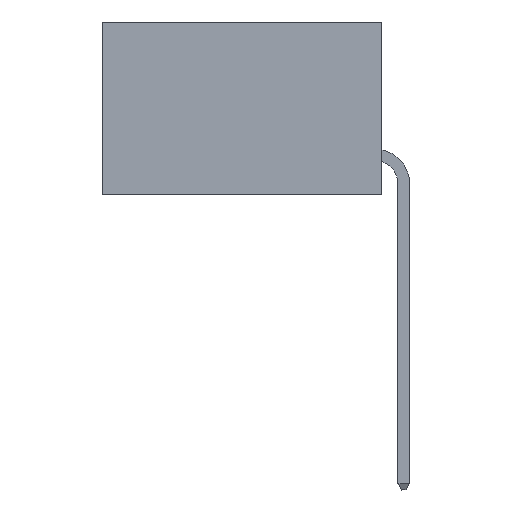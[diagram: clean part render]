
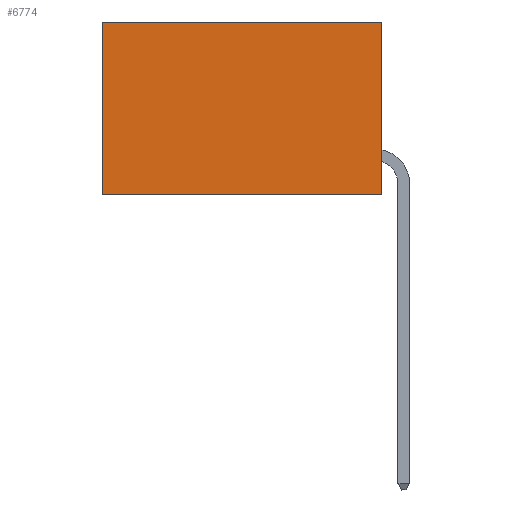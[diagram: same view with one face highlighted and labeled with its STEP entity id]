
A CAD part, left-side view. The second image highlights one B-rep face of the part: STEP entity #6774.
In plain terms, the highlighted planar face has unit normal (-1, 0, 0).
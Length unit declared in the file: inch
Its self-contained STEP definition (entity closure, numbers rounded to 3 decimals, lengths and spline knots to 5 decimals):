
#1500 = VECTOR ( 'NONE', #10096, 39.37008 ) ;
#1621 = CARTESIAN_POINT ( 'NONE',  ( 0.2875, 0.6, 0. ) ) ;
#1684 = CARTESIAN_POINT ( 'NONE',  ( 0.2875, 0., 0. ) ) ;
#2334 = CARTESIAN_POINT ( 'NONE',  ( 0.2875, 0., 0. ) ) ;
#2778 = ORIENTED_EDGE ( 'NONE', *, *, #13709, .F. ) ;
#3225 = DIRECTION ( 'NONE',  ( 0., 0., -1. ) ) ;
#3519 = PLANE ( 'NONE',  #7349 ) ;
#3850 = LINE ( 'NONE', #5357, #6901 ) ;
#4178 = ORIENTED_EDGE ( 'NONE', *, *, #12135, .T. ) ;
#4188 = VERTEX_POINT ( 'NONE', #7121 ) ;
#4254 = EDGE_LOOP ( 'NONE', ( #4178, #9367, #2778, #13090 ) ) ;
#5253 = VECTOR ( 'NONE', #8960, 39.37008 ) ;
#5357 = CARTESIAN_POINT ( 'NONE',  ( 0.2875, 0., 0. ) ) ;
#5642 = CARTESIAN_POINT ( 'NONE',  ( 0.2875, 0., 0. ) ) ;
#5748 = CARTESIAN_POINT ( 'NONE',  ( 0.2875, 0., -0.37 ) ) ;
#6328 = VECTOR ( 'NONE', #7014, 39.37008 ) ;
#6774 = ADVANCED_FACE ( 'NONE', ( #6978 ), #3519, .F. ) ;
#6892 = VERTEX_POINT ( 'NONE', #1684 ) ;
#6901 = VECTOR ( 'NONE', #3225, 39.37008 ) ;
#6978 = FACE_OUTER_BOUND ( 'NONE', #4254, .T. ) ;
#7014 = DIRECTION ( 'NONE',  ( 0., 0., -1. ) ) ;
#7121 = CARTESIAN_POINT ( 'NONE',  ( 0.2875, 0., -0.37 ) ) ;
#7349 = AXIS2_PLACEMENT_3D ( 'NONE', #2334, #12230, #11014 ) ;
#7604 = LINE ( 'NONE', #5748, #1500 ) ;
#8324 = EDGE_CURVE ( 'NONE', #6892, #10423, #13953, .T. ) ;
#8960 = DIRECTION ( 'NONE',  ( 0., 1., 0. ) ) ;
#9367 = ORIENTED_EDGE ( 'NONE', *, *, #13352, .F. ) ;
#9400 = CARTESIAN_POINT ( 'NONE',  ( 0.2875, 0.6, -0.37 ) ) ;
#10096 = DIRECTION ( 'NONE',  ( 0., 1., 0. ) ) ;
#10255 = LINE ( 'NONE', #1621, #6328 ) ;
#10423 = VERTEX_POINT ( 'NONE', #11008 ) ;
#11008 = CARTESIAN_POINT ( 'NONE',  ( 0.2875, 0.6, 0. ) ) ;
#11014 = DIRECTION ( 'NONE',  ( 0., 0., -1. ) ) ;
#11154 = VERTEX_POINT ( 'NONE', #9400 ) ;
#12135 = EDGE_CURVE ( 'NONE', #10423, #11154, #10255, .T. ) ;
#12230 = DIRECTION ( 'NONE',  ( 1., 0., 0. ) ) ;
#13090 = ORIENTED_EDGE ( 'NONE', *, *, #8324, .T. ) ;
#13352 = EDGE_CURVE ( 'NONE', #4188, #11154, #7604, .T. ) ;
#13709 = EDGE_CURVE ( 'NONE', #6892, #4188, #3850, .T. ) ;
#13953 = LINE ( 'NONE', #5642, #5253 ) ;
